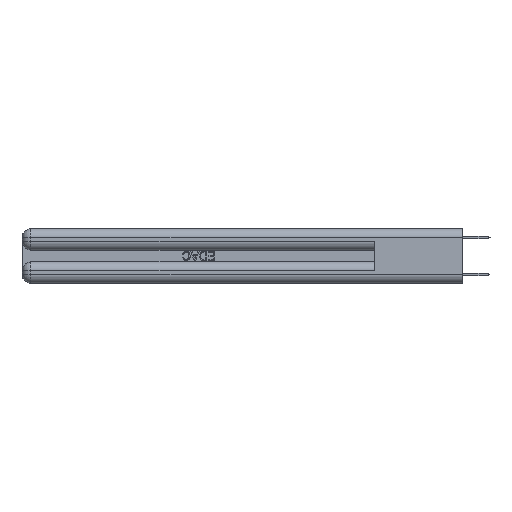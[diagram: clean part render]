
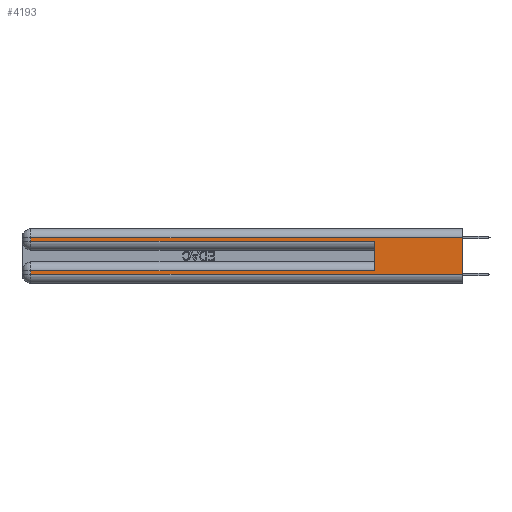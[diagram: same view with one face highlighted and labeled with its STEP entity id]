
A CAD part, left-side view. The second image highlights one B-rep face of the part: STEP entity #4193.
In plain terms, the highlighted planar face has unit normal (-1, 0, 0).
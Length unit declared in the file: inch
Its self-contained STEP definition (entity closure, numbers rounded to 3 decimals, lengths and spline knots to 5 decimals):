
#344 = VECTOR ( 'NONE', #30110, 39.37008 ) ;
#353 = VECTOR ( 'NONE', #13118, 39.37008 ) ;
#805 = LINE ( 'NONE', #7094, #4262 ) ;
#2253 = VERTEX_POINT ( 'NONE', #9730 ) ;
#2467 = VECTOR ( 'NONE', #28217, 39.37008 ) ;
#3048 = CARTESIAN_POINT ( 'NONE',  ( 0., 0.6, 0.145 ) ) ;
#3411 = LINE ( 'NONE', #3048, #344 ) ;
#3608 = VERTEX_POINT ( 'NONE', #14559 ) ;
#4193 = ADVANCED_FACE ( 'NONE', ( #20847 ), #13361, .F. ) ;
#4262 = VECTOR ( 'NONE', #6883, 39.37008 ) ;
#4341 = VERTEX_POINT ( 'NONE', #20925 ) ;
#4394 = ORIENTED_EDGE ( 'NONE', *, *, #21645, .T. ) ;
#4448 = LINE ( 'NONE', #28958, #9421 ) ;
#5922 = DIRECTION ( 'NONE',  ( 0., 0., -1. ) ) ;
#6376 = CARTESIAN_POINT ( 'NONE',  ( 0., 2.94, 0.06 ) ) ;
#6389 = AXIS2_PLACEMENT_3D ( 'NONE', #30416, #20788, #15732 ) ;
#6519 = CARTESIAN_POINT ( 'NONE',  ( 0., 2.94, 0.31 ) ) ;
#6883 = DIRECTION ( 'NONE',  ( 0., 1., 0. ) ) ;
#7054 = EDGE_CURVE ( 'NONE', #14119, #15949, #21486, .T. ) ;
#7094 = CARTESIAN_POINT ( 'NONE',  ( 0., 0., 0.31 ) ) ;
#7804 = EDGE_CURVE ( 'NONE', #24271, #2253, #27502, .T. ) ;
#8332 = VERTEX_POINT ( 'NONE', #15192 ) ;
#9338 = EDGE_CURVE ( 'NONE', #15949, #3608, #4448, .T. ) ;
#9421 = VECTOR ( 'NONE', #24163, 39.37008 ) ;
#9730 = CARTESIAN_POINT ( 'NONE',  ( 0., 0., 0.06 ) ) ;
#11049 = EDGE_CURVE ( 'NONE', #4341, #8332, #24268, .T. ) ;
#11870 = CARTESIAN_POINT ( 'NONE',  ( 0., 2.94, 0.285 ) ) ;
#13118 = DIRECTION ( 'NONE',  ( 0., 0., -1. ) ) ;
#13171 = CARTESIAN_POINT ( 'NONE',  ( 0., 2.94, 0.37 ) ) ;
#13328 = VECTOR ( 'NONE', #24213, 39.37008 ) ;
#13361 = PLANE ( 'NONE',  #6389 ) ;
#13626 = ORIENTED_EDGE ( 'NONE', *, *, #11049, .T. ) ;
#14119 = VERTEX_POINT ( 'NONE', #6519 ) ;
#14340 = VERTEX_POINT ( 'NONE', #6376 ) ;
#14559 = CARTESIAN_POINT ( 'NONE',  ( 0., 0.6, 0.285 ) ) ;
#14702 = CARTESIAN_POINT ( 'NONE',  ( 0., 0., 0.31 ) ) ;
#15192 = CARTESIAN_POINT ( 'NONE',  ( 0., 2.94, 0.085 ) ) ;
#15404 = VECTOR ( 'NONE', #21287, 39.37008 ) ;
#15532 = ORIENTED_EDGE ( 'NONE', *, *, #31158, .F. ) ;
#15732 = DIRECTION ( 'NONE',  ( 0., 0., -1. ) ) ;
#15949 = VERTEX_POINT ( 'NONE', #11870 ) ;
#17069 = EDGE_CURVE ( 'NONE', #24271, #14119, #805, .T. ) ;
#17966 = CARTESIAN_POINT ( 'NONE',  ( 0., 0., 0.37 ) ) ;
#18031 = VECTOR ( 'NONE', #5922, 39.37008 ) ;
#18959 = CARTESIAN_POINT ( 'NONE',  ( 0., 0., 0.085 ) ) ;
#19707 = CARTESIAN_POINT ( 'NONE',  ( 0., 0., 0.06 ) ) ;
#20788 = DIRECTION ( 'NONE',  ( 1., 0., 0. ) ) ;
#20847 = FACE_OUTER_BOUND ( 'NONE', #28967, .T. ) ;
#20925 = CARTESIAN_POINT ( 'NONE',  ( 0., 0.6, 0.085 ) ) ;
#21265 = CARTESIAN_POINT ( 'NONE',  ( 0., 2.94, 0.37 ) ) ;
#21287 = DIRECTION ( 'NONE',  ( 0., 1., 0. ) ) ;
#21486 = LINE ( 'NONE', #13171, #18031 ) ;
#21645 = EDGE_CURVE ( 'NONE', #14340, #2253, #26409, .T. ) ;
#22011 = LINE ( 'NONE', #21265, #2467 ) ;
#22365 = ORIENTED_EDGE ( 'NONE', *, *, #9338, .T. ) ;
#23039 = EDGE_CURVE ( 'NONE', #8332, #14340, #22011, .T. ) ;
#23482 = ORIENTED_EDGE ( 'NONE', *, *, #23039, .T. ) ;
#24163 = DIRECTION ( 'NONE',  ( 0., -1., 0. ) ) ;
#24213 = DIRECTION ( 'NONE',  ( 0., -1., 0. ) ) ;
#24268 = LINE ( 'NONE', #18959, #15404 ) ;
#24271 = VERTEX_POINT ( 'NONE', #14702 ) ;
#26409 = LINE ( 'NONE', #19707, #13328 ) ;
#27502 = LINE ( 'NONE', #17966, #353 ) ;
#28217 = DIRECTION ( 'NONE',  ( 0., 0., -1. ) ) ;
#28958 = CARTESIAN_POINT ( 'NONE',  ( 0., 0., 0.285 ) ) ;
#28967 = EDGE_LOOP ( 'NONE', ( #30532, #29132, #30985, #22365, #15532, #13626, #23482, #4394 ) ) ;
#29132 = ORIENTED_EDGE ( 'NONE', *, *, #17069, .T. ) ;
#30110 = DIRECTION ( 'NONE',  ( 0., 0., 1. ) ) ;
#30416 = CARTESIAN_POINT ( 'NONE',  ( 0., 0., 0.37 ) ) ;
#30532 = ORIENTED_EDGE ( 'NONE', *, *, #7804, .F. ) ;
#30985 = ORIENTED_EDGE ( 'NONE', *, *, #7054, .T. ) ;
#31158 = EDGE_CURVE ( 'NONE', #4341, #3608, #3411, .T. ) ;
